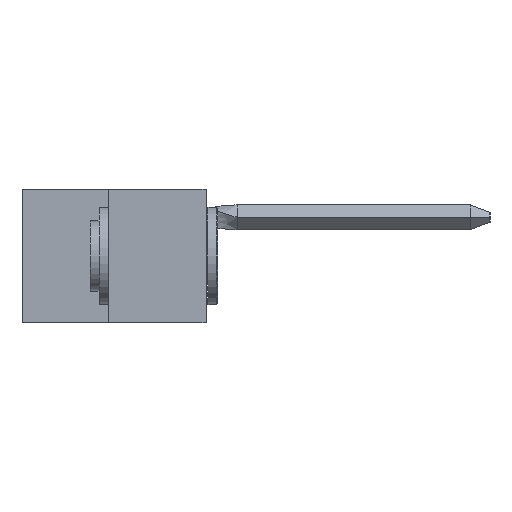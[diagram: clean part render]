
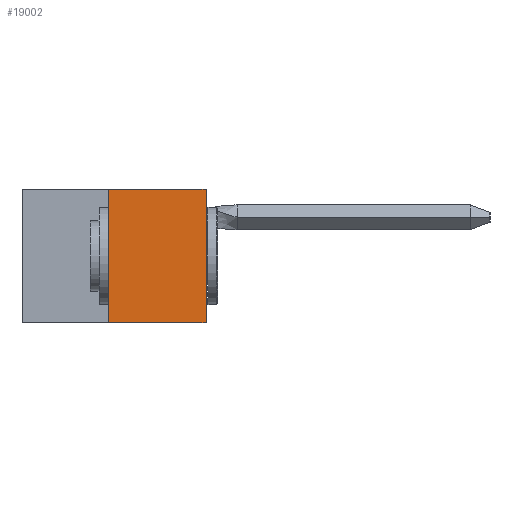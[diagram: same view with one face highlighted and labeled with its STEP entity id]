
A CAD part, left-side view. The second image highlights one B-rep face of the part: STEP entity #19002.
In plain terms, the highlighted planar face has unit normal (-1, 0, 0).
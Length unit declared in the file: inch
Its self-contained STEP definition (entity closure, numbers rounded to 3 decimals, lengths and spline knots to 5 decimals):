
#385 = DIRECTION ( 'NONE',  ( 0., 0., 1. ) ) ;
#737 = VECTOR ( 'NONE', #385, 39.37008 ) ;
#821 = CARTESIAN_POINT ( 'NONE',  ( 0., 0.473, 0. ) ) ;
#1231 = VECTOR ( 'NONE', #3807, 39.37008 ) ;
#1368 = ORIENTED_EDGE ( 'NONE', *, *, #32992, .T. ) ;
#2001 = AXIS2_PLACEMENT_3D ( 'NONE', #821, #24720, #33316 ) ;
#3807 = DIRECTION ( 'NONE',  ( 0., -1., 0. ) ) ;
#4105 = PLANE ( 'NONE',  #2001 ) ;
#4741 = FACE_OUTER_BOUND ( 'NONE', #28892, .T. ) ;
#4788 = VECTOR ( 'NONE', #20107, 39.37008 ) ;
#9038 = VERTEX_POINT ( 'NONE', #28883 ) ;
#12188 = CARTESIAN_POINT ( 'NONE',  ( 0., 0., 0. ) ) ;
#14179 = CARTESIAN_POINT ( 'NONE',  ( 0., 0.473, -0.343 ) ) ;
#16902 = LINE ( 'NONE', #18501, #1231 ) ;
#18001 = ORIENTED_EDGE ( 'NONE', *, *, #31987, .F. ) ;
#18501 = CARTESIAN_POINT ( 'NONE',  ( 0., 0.473, 0. ) ) ;
#19002 = ADVANCED_FACE ( 'NONE', ( #4741 ), #4105, .F. ) ;
#20107 = DIRECTION ( 'NONE',  ( 0., -1., 0. ) ) ;
#20452 = LINE ( 'NONE', #14179, #4788 ) ;
#21798 = VERTEX_POINT ( 'NONE', #27821 ) ;
#22112 = CARTESIAN_POINT ( 'NONE',  ( 0., 0.25, 0. ) ) ;
#24720 = DIRECTION ( 'NONE',  ( 1., 0., 0. ) ) ;
#25098 = DIRECTION ( 'NONE',  ( 0., 0., 1. ) ) ;
#26979 = VERTEX_POINT ( 'NONE', #35214 ) ;
#27692 = ORIENTED_EDGE ( 'NONE', *, *, #35246, .F. ) ;
#27821 = CARTESIAN_POINT ( 'NONE',  ( 0., 0.25, -0.343 ) ) ;
#28883 = CARTESIAN_POINT ( 'NONE',  ( 0., 0.25, 0. ) ) ;
#28892 = EDGE_LOOP ( 'NONE', ( #18001, #27692, #1368, #30688 ) ) ;
#29219 = LINE ( 'NONE', #12188, #737 ) ;
#29316 = CARTESIAN_POINT ( 'NONE',  ( 0., 0., -0.343 ) ) ;
#30260 = VECTOR ( 'NONE', #25098, 39.37008 ) ;
#30688 = ORIENTED_EDGE ( 'NONE', *, *, #37617, .T. ) ;
#31430 = VERTEX_POINT ( 'NONE', #29316 ) ;
#31987 = EDGE_CURVE ( 'NONE', #9038, #26979, #16902, .T. ) ;
#32992 = EDGE_CURVE ( 'NONE', #21798, #31430, #20452, .T. ) ;
#33316 = DIRECTION ( 'NONE',  ( 0., 0., -1. ) ) ;
#35214 = CARTESIAN_POINT ( 'NONE',  ( 0., 0., 0. ) ) ;
#35246 = EDGE_CURVE ( 'NONE', #21798, #9038, #35780, .T. ) ;
#35780 = LINE ( 'NONE', #22112, #30260 ) ;
#37617 = EDGE_CURVE ( 'NONE', #31430, #26979, #29219, .T. ) ;
